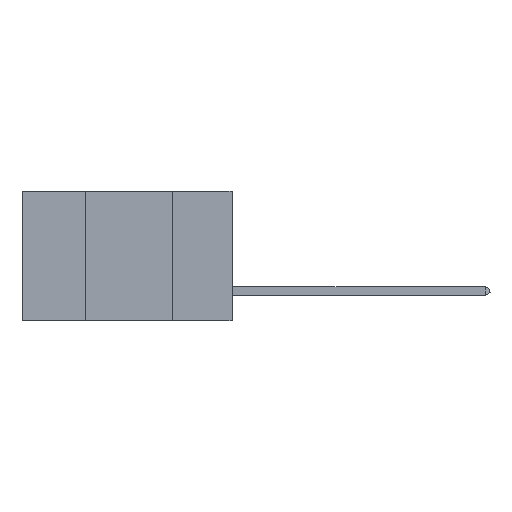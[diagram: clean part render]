
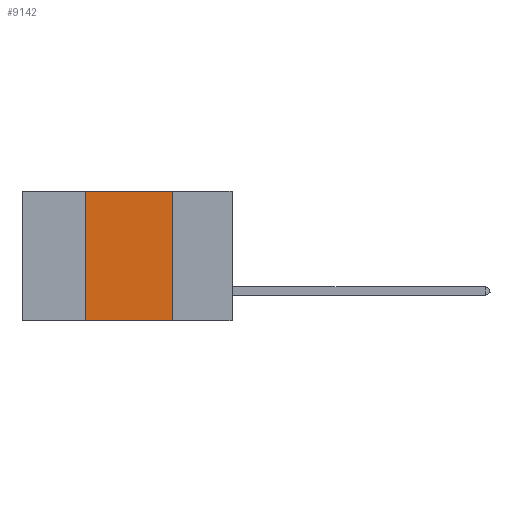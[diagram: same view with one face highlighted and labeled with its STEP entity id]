
A CAD part, left-side view. The second image highlights one B-rep face of the part: STEP entity #9142.
In plain terms, the highlighted planar face has unit normal (-1, 0, 0).
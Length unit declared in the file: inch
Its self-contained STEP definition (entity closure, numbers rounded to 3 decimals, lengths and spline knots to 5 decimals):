
#117 = EDGE_LOOP ( 'NONE', ( #4056, #4492, #12864, #2555 ) ) ;
#728 = VERTEX_POINT ( 'NONE', #11194 ) ;
#1568 = DIRECTION ( 'NONE',  ( 0., -1., 0. ) ) ;
#2555 = ORIENTED_EDGE ( 'NONE', *, *, #9290, .T. ) ;
#3747 = VECTOR ( 'NONE', #1568, 39.37008 ) ;
#4056 = ORIENTED_EDGE ( 'NONE', *, *, #8394, .F. ) ;
#4492 = ORIENTED_EDGE ( 'NONE', *, *, #13189, .F. ) ;
#5452 = DIRECTION ( 'NONE',  ( 0., -1., 0. ) ) ;
#5945 = CARTESIAN_POINT ( 'NONE',  ( 0., 0.17, 0. ) ) ;
#6661 = CARTESIAN_POINT ( 'NONE',  ( 0., 0.6, -0.37 ) ) ;
#7316 = EDGE_CURVE ( 'NONE', #728, #14534, #12885, .T. ) ;
#7417 = LINE ( 'NONE', #11363, #3747 ) ;
#7548 = VECTOR ( 'NONE', #14044, 39.37008 ) ;
#7889 = VECTOR ( 'NONE', #13776, 39.37008 ) ;
#7953 = CARTESIAN_POINT ( 'NONE',  ( 0., 0.6, 0. ) ) ;
#8286 = CARTESIAN_POINT ( 'NONE',  ( 0., 0.42, 0. ) ) ;
#8394 = EDGE_CURVE ( 'NONE', #15160, #8689, #14464, .T. ) ;
#8689 = VERTEX_POINT ( 'NONE', #15114 ) ;
#9142 = ADVANCED_FACE ( 'NONE', ( #9454 ), #10723, .F. ) ;
#9290 = EDGE_CURVE ( 'NONE', #728, #8689, #15347, .T. ) ;
#9454 = FACE_OUTER_BOUND ( 'NONE', #117, .T. ) ;
#10723 = PLANE ( 'NONE',  #11223 ) ;
#11194 = CARTESIAN_POINT ( 'NONE',  ( 0., 0.42, -0.37 ) ) ;
#11223 = AXIS2_PLACEMENT_3D ( 'NONE', #7953, #12176, #16425 ) ;
#11363 = CARTESIAN_POINT ( 'NONE',  ( 0., 0.6, 0. ) ) ;
#12176 = DIRECTION ( 'NONE',  ( 1., 0., 0. ) ) ;
#12363 = CARTESIAN_POINT ( 'NONE',  ( 0., 0.17, 0. ) ) ;
#12864 = ORIENTED_EDGE ( 'NONE', *, *, #7316, .F. ) ;
#12885 = LINE ( 'NONE', #14742, #7889 ) ;
#13189 = EDGE_CURVE ( 'NONE', #14534, #15160, #7417, .T. ) ;
#13776 = DIRECTION ( 'NONE',  ( 0., 0., 1. ) ) ;
#14044 = DIRECTION ( 'NONE',  ( 0., 0., -1. ) ) ;
#14464 = LINE ( 'NONE', #5945, #7548 ) ;
#14534 = VERTEX_POINT ( 'NONE', #8286 ) ;
#14742 = CARTESIAN_POINT ( 'NONE',  ( 0., 0.42, 0. ) ) ;
#15114 = CARTESIAN_POINT ( 'NONE',  ( 0., 0.17, -0.37 ) ) ;
#15160 = VERTEX_POINT ( 'NONE', #12363 ) ;
#15347 = LINE ( 'NONE', #6661, #17281 ) ;
#16425 = DIRECTION ( 'NONE',  ( 0., 0., -1. ) ) ;
#17281 = VECTOR ( 'NONE', #5452, 39.37008 ) ;
